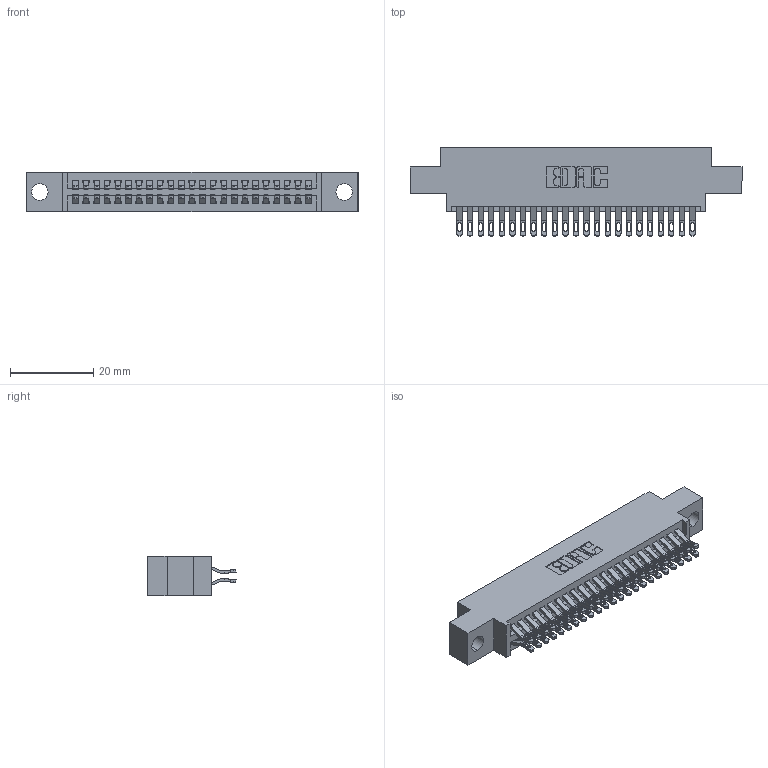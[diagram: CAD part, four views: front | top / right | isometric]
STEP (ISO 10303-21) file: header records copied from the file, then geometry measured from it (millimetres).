
FILE_DESCRIPTION (( 'STEP AP203' ), '1' );
FILE_NAME ('395-046-555-804.STEP', '2021-06-16T23:09:54', ( '' ), ( '' ), 'SwSTEP 2.0', 'SolidWorks 2020', '' );
FILE_SCHEMA (( 'CONFIG_CONTROL_DESIGN' ));
Length unit declared in the file: inch
Products named in the file (3): 345-292-001_555 Tail; 345 Part_0.170 Offset - 0.156 Dia-TI; 395-046-555-804
Assembly tree (47 placements, depth 2):
  395-046-555-804
    345 Part_0.170 Offset - 0.156 Dia-TI
    345-292-001_555 Tail  x46
Bounding box: 79.63 x 21.13 x 9.4 mm (x, y, z)
Volume: 7473 mm3; surface area: 11137.4 mm2
Topology: 47 solids, 47 shells, 2720 faces, 8531 edges, 5686 vertices
Faces by surface type: plane 1524, cylinder 1196
Entity records: 21481 total; most frequent: CARTESIAN_POINT 3660, ORIENTED_EDGE 3562, DIRECTION 3217, EDGE_CURVE 1781, VECTOR 1537, LINE 1537, VERTEX_POINT 1186, AXIS2_PLACEMENT_3D 840
